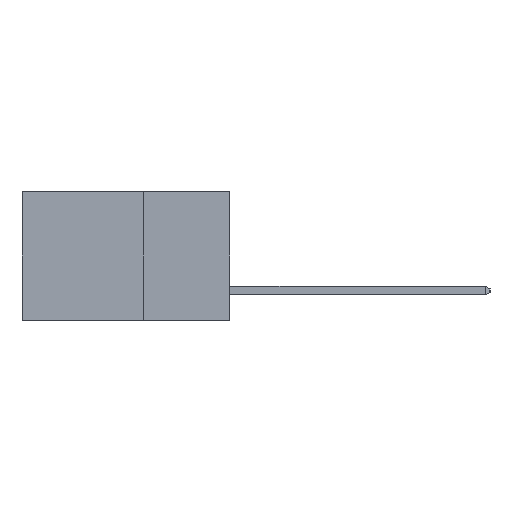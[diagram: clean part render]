
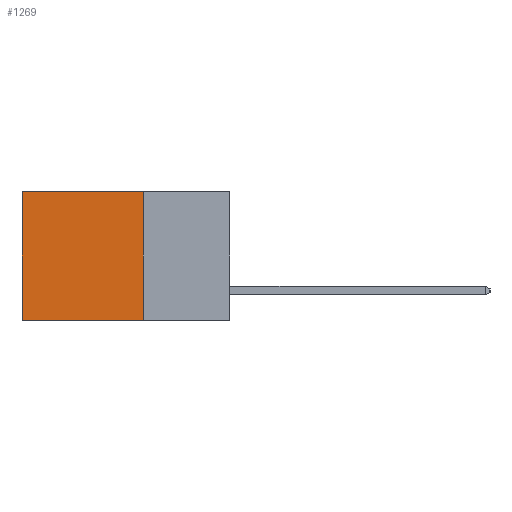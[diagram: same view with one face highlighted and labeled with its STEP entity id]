
A CAD part, left-side view. The second image highlights one B-rep face of the part: STEP entity #1269.
In plain terms, the highlighted planar face has unit normal (-1, 0, 0).
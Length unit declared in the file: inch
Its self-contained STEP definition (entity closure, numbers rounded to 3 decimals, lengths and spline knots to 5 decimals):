
#313 = ORIENTED_EDGE ( 'NONE', *, *, #3078, .F. ) ;
#406 = CARTESIAN_POINT ( 'NONE',  ( 0.298, 0.25, -0.37 ) ) ;
#1269 = ADVANCED_FACE ( 'NONE', ( #9140 ), #3462, .F. ) ;
#1454 = VERTEX_POINT ( 'NONE', #406 ) ;
#2280 = LINE ( 'NONE', #9677, #6708 ) ;
#2396 = DIRECTION ( 'NONE',  ( 1., 0., 0. ) ) ;
#2572 = VERTEX_POINT ( 'NONE', #10001 ) ;
#2595 = DIRECTION ( 'NONE',  ( 0., 0., -1. ) ) ;
#3078 = EDGE_CURVE ( 'NONE', #1454, #4762, #15437, .T. ) ;
#3462 = PLANE ( 'NONE',  #9634 ) ;
#3549 = CARTESIAN_POINT ( 'NONE',  ( 0.298, 0.25, 0. ) ) ;
#4564 = VECTOR ( 'NONE', #6907, 39.37008 ) ;
#4762 = VERTEX_POINT ( 'NONE', #14647 ) ;
#6708 = VECTOR ( 'NONE', #14471, 39.37008 ) ;
#6907 = DIRECTION ( 'NONE',  ( 0., 0., -1. ) ) ;
#7046 = ORIENTED_EDGE ( 'NONE', *, *, #8286, .T. ) ;
#7773 = CARTESIAN_POINT ( 'NONE',  ( 0.298, 0.25, -0.37 ) ) ;
#8286 = EDGE_CURVE ( 'NONE', #2572, #9480, #2280, .T. ) ;
#8709 = DIRECTION ( 'NONE',  ( 0., 1., 0. ) ) ;
#9140 = FACE_OUTER_BOUND ( 'NONE', #14604, .T. ) ;
#9480 = VERTEX_POINT ( 'NONE', #16221 ) ;
#9634 = AXIS2_PLACEMENT_3D ( 'NONE', #3549, #2396, #2595 ) ;
#9677 = CARTESIAN_POINT ( 'NONE',  ( 0.298, 0.25, 0. ) ) ;
#10001 = CARTESIAN_POINT ( 'NONE',  ( 0.298, 0.25, 0. ) ) ;
#10536 = EDGE_CURVE ( 'NONE', #9480, #4762, #16294, .T. ) ;
#12317 = VECTOR ( 'NONE', #8709, 39.37008 ) ;
#12479 = VECTOR ( 'NONE', #15907, 39.37008 ) ;
#13013 = ORIENTED_EDGE ( 'NONE', *, *, #14207, .F. ) ;
#14144 = CARTESIAN_POINT ( 'NONE',  ( 0.298, 0.25, 0. ) ) ;
#14207 = EDGE_CURVE ( 'NONE', #2572, #1454, #14319, .T. ) ;
#14319 = LINE ( 'NONE', #14144, #4564 ) ;
#14471 = DIRECTION ( 'NONE',  ( 0., 1., 0. ) ) ;
#14604 = EDGE_LOOP ( 'NONE', ( #15930, #313, #13013, #7046 ) ) ;
#14647 = CARTESIAN_POINT ( 'NONE',  ( 0.298, 0.6, -0.37 ) ) ;
#14703 = CARTESIAN_POINT ( 'NONE',  ( 0.298, 0.6, 0. ) ) ;
#15437 = LINE ( 'NONE', #7773, #12317 ) ;
#15907 = DIRECTION ( 'NONE',  ( 0., 0., -1. ) ) ;
#15930 = ORIENTED_EDGE ( 'NONE', *, *, #10536, .T. ) ;
#16221 = CARTESIAN_POINT ( 'NONE',  ( 0.298, 0.6, 0. ) ) ;
#16294 = LINE ( 'NONE', #14703, #12479 ) ;
